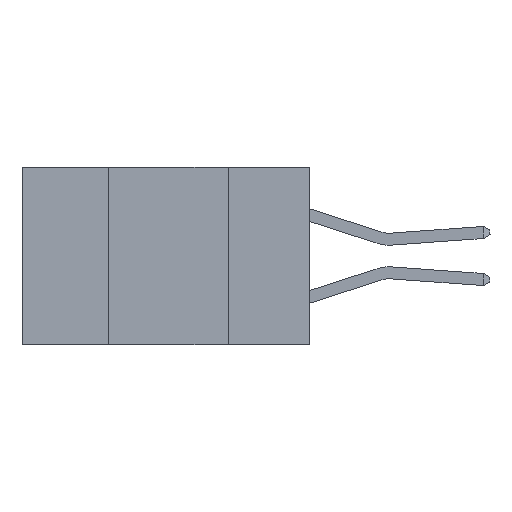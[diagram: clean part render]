
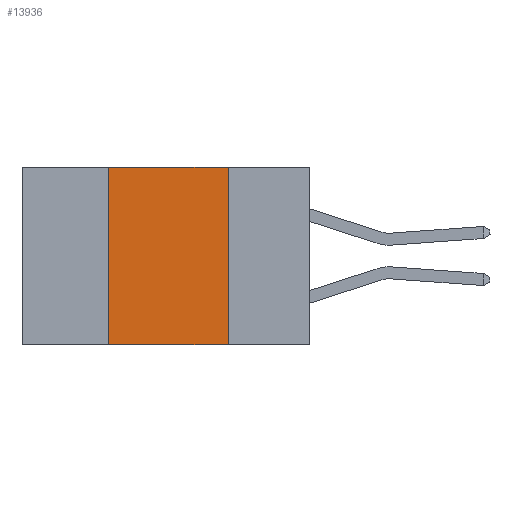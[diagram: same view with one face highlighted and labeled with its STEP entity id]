
A CAD part, left-side view. The second image highlights one B-rep face of the part: STEP entity #13936.
In plain terms, the highlighted planar face has unit normal (-1, 0, 0).
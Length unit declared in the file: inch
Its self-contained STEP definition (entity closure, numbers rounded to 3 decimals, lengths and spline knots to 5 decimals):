
#1124 = EDGE_CURVE ( 'NONE', #2754, #2685, #8883, .T. ) ;
#2685 = VERTEX_POINT ( 'NONE', #20862 ) ;
#2754 = VERTEX_POINT ( 'NONE', #24432 ) ;
#3077 = VECTOR ( 'NONE', #17240, 39.37008 ) ;
#3168 = VERTEX_POINT ( 'NONE', #9221 ) ;
#3239 = DIRECTION ( 'NONE',  ( 1., 0., 0. ) ) ;
#3668 = VECTOR ( 'NONE', #6814, 39.37008 ) ;
#4605 = LINE ( 'NONE', #18304, #5895 ) ;
#5895 = VECTOR ( 'NONE', #8586, 39.37008 ) ;
#6060 = VERTEX_POINT ( 'NONE', #15571 ) ;
#6814 = DIRECTION ( 'NONE',  ( 0., 0., -1. ) ) ;
#7333 = DIRECTION ( 'NONE',  ( 0., 0., 1. ) ) ;
#7338 = CARTESIAN_POINT ( 'NONE',  ( 0., 0.17, -0.37 ) ) ;
#8165 = EDGE_CURVE ( 'NONE', #2754, #3168, #15910, .T. ) ;
#8586 = DIRECTION ( 'NONE',  ( 0., -1., 0. ) ) ;
#8883 = LINE ( 'NONE', #24828, #21417 ) ;
#9221 = CARTESIAN_POINT ( 'NONE',  ( 0., 0.17, -0.37 ) ) ;
#11205 = PLANE ( 'NONE',  #17741 ) ;
#13330 = ORIENTED_EDGE ( 'NONE', *, *, #8165, .T. ) ;
#13936 = ADVANCED_FACE ( 'NONE', ( #24602 ), #11205, .F. ) ;
#14538 = ORIENTED_EDGE ( 'NONE', *, *, #22003, .F. ) ;
#15571 = CARTESIAN_POINT ( 'NONE',  ( 0., 0.17, 0. ) ) ;
#15910 = LINE ( 'NONE', #20802, #3077 ) ;
#17088 = LINE ( 'NONE', #7338, #3668 ) ;
#17240 = DIRECTION ( 'NONE',  ( 0., -1., 0. ) ) ;
#17741 = AXIS2_PLACEMENT_3D ( 'NONE', #22933, #3239, #21034 ) ;
#18304 = CARTESIAN_POINT ( 'NONE',  ( 0., 0.6, 0. ) ) ;
#19873 = ORIENTED_EDGE ( 'NONE', *, *, #1124, .F. ) ;
#20802 = CARTESIAN_POINT ( 'NONE',  ( 0., 0.6, -0.37 ) ) ;
#20862 = CARTESIAN_POINT ( 'NONE',  ( 0., 0.42, 0. ) ) ;
#21034 = DIRECTION ( 'NONE',  ( 0., 0., -1. ) ) ;
#21173 = EDGE_CURVE ( 'NONE', #2685, #6060, #4605, .T. ) ;
#21417 = VECTOR ( 'NONE', #7333, 39.37008 ) ;
#22003 = EDGE_CURVE ( 'NONE', #6060, #3168, #17088, .T. ) ;
#22023 = ORIENTED_EDGE ( 'NONE', *, *, #21173, .F. ) ;
#22933 = CARTESIAN_POINT ( 'NONE',  ( 0., 0.6, 0. ) ) ;
#23122 = EDGE_LOOP ( 'NONE', ( #14538, #22023, #19873, #13330 ) ) ;
#24432 = CARTESIAN_POINT ( 'NONE',  ( 0., 0.42, -0.37 ) ) ;
#24602 = FACE_OUTER_BOUND ( 'NONE', #23122, .T. ) ;
#24828 = CARTESIAN_POINT ( 'NONE',  ( 0., 0.42, -0.37 ) ) ;
